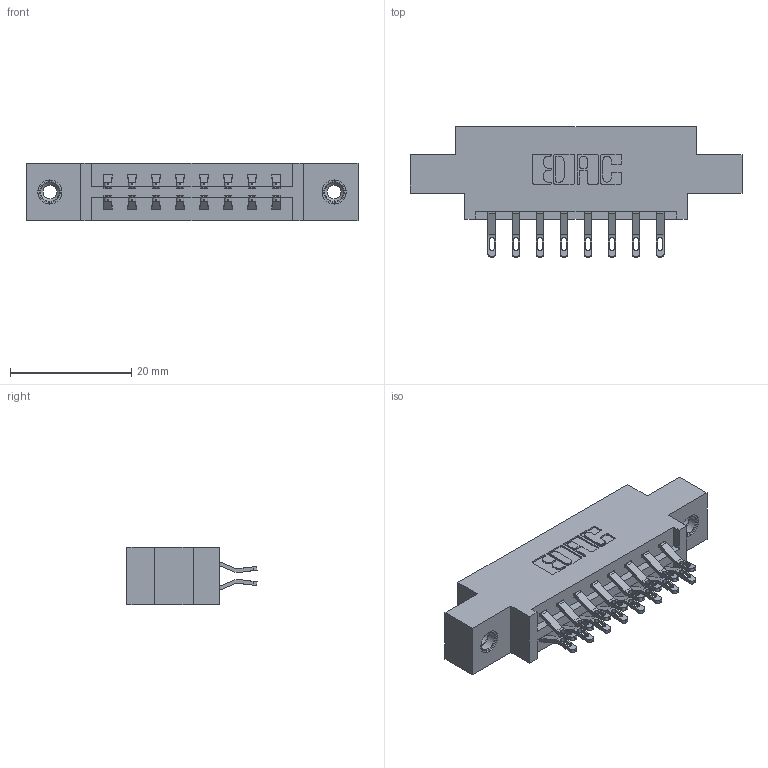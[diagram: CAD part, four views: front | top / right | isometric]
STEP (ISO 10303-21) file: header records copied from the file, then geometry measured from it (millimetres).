
FILE_DESCRIPTION (( 'STEP AP203' ), '1' );
FILE_NAME ('337-016-555-808.STEP', '2018-08-04T20:15:22', ( '' ), ( '' ), 'SwSTEP 2.0', 'SolidWorks 2016', '' );
FILE_SCHEMA (( 'CONFIG_CONTROL_DESIGN' ));
Length unit declared in the file: inch
Products named in the file (4): 337 Part_0.170 Offset - 0.156 Dia-TI; 345-292-001_555 Tail; 345-250-001_345-250-003-102; 337-016-555-808
Assembly tree (19 placements, depth 2):
  337-016-555-808
    337 Part_0.170 Offset - 0.156 Dia-TI
    345-292-001_555 Tail  x16
    345-250-001_345-250-003-102  x2
Bounding box: 54.71 x 21.47 x 9.4 mm (x, y, z)
Volume: 5235.8 mm3; surface area: 5895.4 mm2
Topology: 19 solids, 19 shells, 1138 faces, 3483 edges, 2314 vertices
Faces by surface type: plane 682, cylinder 440, cone 12, torus 4
Entity records: 12244 total; most frequent: CARTESIAN_POINT 2107, ORIENTED_EDGE 2006, DIRECTION 1857, EDGE_CURVE 1003, LINE 835, VECTOR 835, VERTEX_POINT 664, AXIS2_PLACEMENT_3D 511
